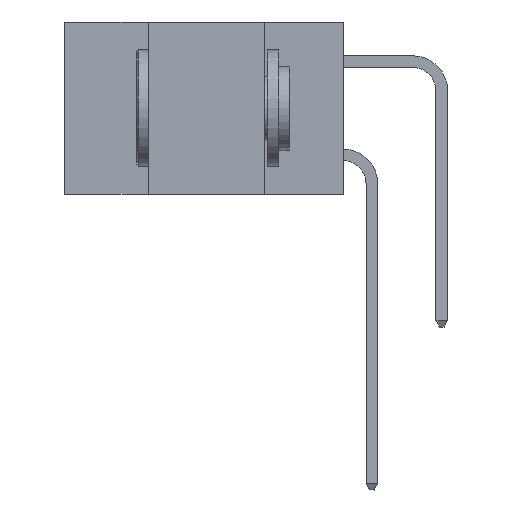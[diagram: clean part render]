
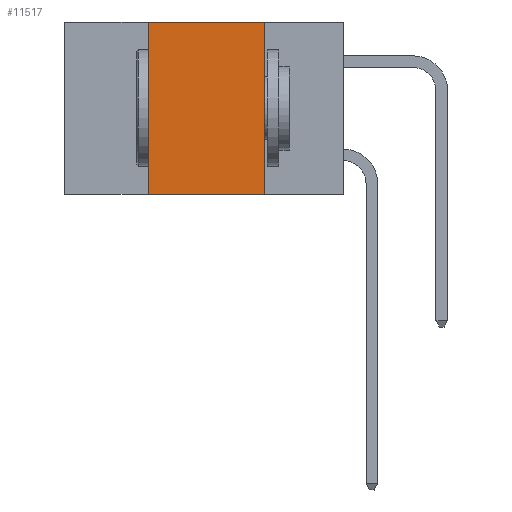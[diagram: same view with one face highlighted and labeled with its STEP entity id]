
A CAD part, left-side view. The second image highlights one B-rep face of the part: STEP entity #11517.
In plain terms, the highlighted planar face has unit normal (-1, 0, 0).
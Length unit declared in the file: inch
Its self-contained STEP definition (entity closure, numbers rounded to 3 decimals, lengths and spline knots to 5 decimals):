
#1783 = DIRECTION ( 'NONE',  ( 0., 0., -1. ) ) ;
#2255 = EDGE_LOOP ( 'NONE', ( #11646, #11971, #5385, #13466 ) ) ;
#2564 = VERTEX_POINT ( 'NONE', #12271 ) ;
#2751 = CARTESIAN_POINT ( 'NONE',  ( 0., 0.6, -0.37 ) ) ;
#3010 = VERTEX_POINT ( 'NONE', #10509 ) ;
#3067 = CARTESIAN_POINT ( 'NONE',  ( 0., 0.6, 0. ) ) ;
#3833 = DIRECTION ( 'NONE',  ( 0., -1., 0. ) ) ;
#3843 = CARTESIAN_POINT ( 'NONE',  ( 0., 0.17, 0. ) ) ;
#4048 = CARTESIAN_POINT ( 'NONE',  ( 0., 0.6, 0. ) ) ;
#4114 = FACE_OUTER_BOUND ( 'NONE', #2255, .T. ) ;
#4192 = LINE ( 'NONE', #3843, #13942 ) ;
#5008 = LINE ( 'NONE', #3067, #13289 ) ;
#5385 = ORIENTED_EDGE ( 'NONE', *, *, #13756, .F. ) ;
#5693 = VECTOR ( 'NONE', #15019, 39.37008 ) ;
#6174 = CARTESIAN_POINT ( 'NONE',  ( 0., 0.17, 0. ) ) ;
#6516 = PLANE ( 'NONE',  #7482 ) ;
#6748 = CARTESIAN_POINT ( 'NONE',  ( 0., 0.42, 0. ) ) ;
#7482 = AXIS2_PLACEMENT_3D ( 'NONE', #4048, #14624, #1783 ) ;
#7815 = LINE ( 'NONE', #2751, #13550 ) ;
#8997 = LINE ( 'NONE', #6748, #5693 ) ;
#9029 = EDGE_CURVE ( 'NONE', #14241, #3010, #4192, .T. ) ;
#9494 = DIRECTION ( 'NONE',  ( 0., 0., -1. ) ) ;
#10416 = EDGE_CURVE ( 'NONE', #2564, #3010, #7815, .T. ) ;
#10509 = CARTESIAN_POINT ( 'NONE',  ( 0., 0.17, -0.37 ) ) ;
#11517 = ADVANCED_FACE ( 'NONE', ( #4114 ), #6516, .F. ) ;
#11646 = ORIENTED_EDGE ( 'NONE', *, *, #9029, .F. ) ;
#11971 = ORIENTED_EDGE ( 'NONE', *, *, #12357, .F. ) ;
#12271 = CARTESIAN_POINT ( 'NONE',  ( 0., 0.42, -0.37 ) ) ;
#12357 = EDGE_CURVE ( 'NONE', #14084, #14241, #5008, .T. ) ;
#13289 = VECTOR ( 'NONE', #14854, 39.37008 ) ;
#13466 = ORIENTED_EDGE ( 'NONE', *, *, #10416, .T. ) ;
#13518 = CARTESIAN_POINT ( 'NONE',  ( 0., 0.42, 0. ) ) ;
#13550 = VECTOR ( 'NONE', #3833, 39.37008 ) ;
#13756 = EDGE_CURVE ( 'NONE', #2564, #14084, #8997, .T. ) ;
#13942 = VECTOR ( 'NONE', #9494, 39.37008 ) ;
#14084 = VERTEX_POINT ( 'NONE', #13518 ) ;
#14241 = VERTEX_POINT ( 'NONE', #6174 ) ;
#14624 = DIRECTION ( 'NONE',  ( 1., 0., 0. ) ) ;
#14854 = DIRECTION ( 'NONE',  ( 0., -1., 0. ) ) ;
#15019 = DIRECTION ( 'NONE',  ( 0., 0., 1. ) ) ;
